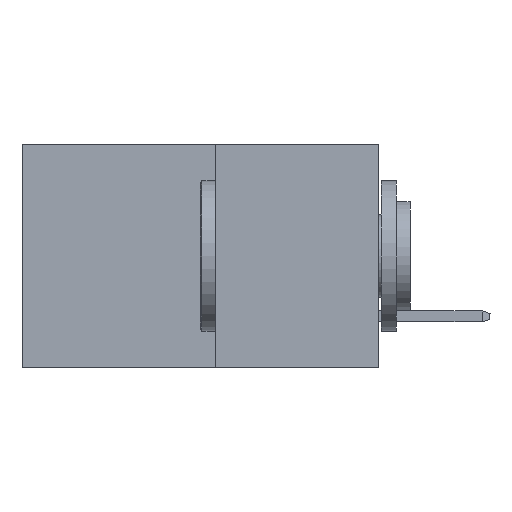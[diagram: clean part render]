
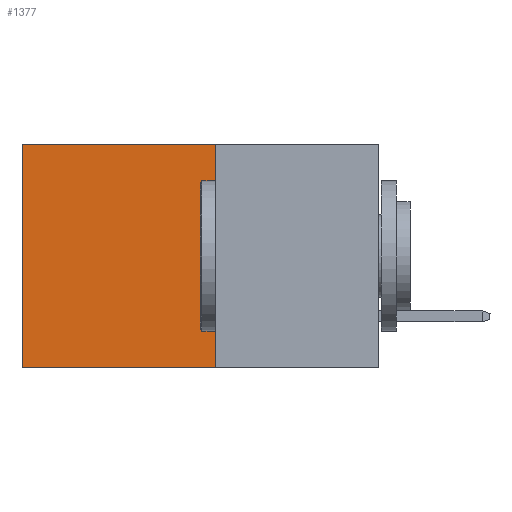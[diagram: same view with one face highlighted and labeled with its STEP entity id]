
A CAD part, left-side view. The second image highlights one B-rep face of the part: STEP entity #1377.
In plain terms, the highlighted planar face has unit normal (-1, 0, 0).
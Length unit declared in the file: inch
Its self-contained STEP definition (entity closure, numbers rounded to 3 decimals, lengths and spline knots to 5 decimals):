
#153 = CARTESIAN_POINT ( 'NONE',  ( 0.277, 0.27, 0. ) ) ;
#684 = VECTOR ( 'NONE', #2647, 39.37008 ) ;
#1377 = ADVANCED_FACE ( 'NONE', ( #27120 ), #6733, .F. ) ;
#1593 = ORIENTED_EDGE ( 'NONE', *, *, #11115, .T. ) ;
#1860 = CARTESIAN_POINT ( 'NONE',  ( 0.277, 0.27, 0. ) ) ;
#2647 = DIRECTION ( 'NONE',  ( 0., 1., 0. ) ) ;
#4749 = VERTEX_POINT ( 'NONE', #24941 ) ;
#5170 = CARTESIAN_POINT ( 'NONE',  ( 0.277, 0.27, -0.37 ) ) ;
#5468 = LINE ( 'NONE', #20682, #18034 ) ;
#6733 = PLANE ( 'NONE',  #15053 ) ;
#8735 = CARTESIAN_POINT ( 'NONE',  ( 0.277, 0.59, -0.37 ) ) ;
#9065 = DIRECTION ( 'NONE',  ( 1., 0., 0. ) ) ;
#9703 = LINE ( 'NONE', #17524, #22224 ) ;
#11115 = EDGE_CURVE ( 'NONE', #4749, #25093, #28056, .T. ) ;
#13111 = VECTOR ( 'NONE', #19176, 39.37008 ) ;
#14018 = LINE ( 'NONE', #153, #684 ) ;
#15053 = AXIS2_PLACEMENT_3D ( 'NONE', #5170, #9065, #28737 ) ;
#15394 = DIRECTION ( 'NONE',  ( 0., 1., 0. ) ) ;
#17524 = CARTESIAN_POINT ( 'NONE',  ( 0.277, 0.27, -0.37 ) ) ;
#18034 = VECTOR ( 'NONE', #18141, 39.37008 ) ;
#18141 = DIRECTION ( 'NONE',  ( 0., 0., -1. ) ) ;
#19176 = DIRECTION ( 'NONE',  ( 0., 0., -1. ) ) ;
#19711 = EDGE_CURVE ( 'NONE', #22144, #25093, #9703, .T. ) ;
#20682 = CARTESIAN_POINT ( 'NONE',  ( 0.277, 0.27, -0.37 ) ) ;
#21290 = ORIENTED_EDGE ( 'NONE', *, *, #19711, .F. ) ;
#22144 = VERTEX_POINT ( 'NONE', #28271 ) ;
#22224 = VECTOR ( 'NONE', #15394, 39.37008 ) ;
#23909 = EDGE_CURVE ( 'NONE', #28597, #22144, #5468, .T. ) ;
#24930 = EDGE_CURVE ( 'NONE', #28597, #4749, #14018, .T. ) ;
#24941 = CARTESIAN_POINT ( 'NONE',  ( 0.277, 0.59, 0. ) ) ;
#25093 = VERTEX_POINT ( 'NONE', #28472 ) ;
#25309 = EDGE_LOOP ( 'NONE', ( #1593, #21290, #27329, #26230 ) ) ;
#26230 = ORIENTED_EDGE ( 'NONE', *, *, #24930, .T. ) ;
#27120 = FACE_OUTER_BOUND ( 'NONE', #25309, .T. ) ;
#27329 = ORIENTED_EDGE ( 'NONE', *, *, #23909, .F. ) ;
#28056 = LINE ( 'NONE', #8735, #13111 ) ;
#28271 = CARTESIAN_POINT ( 'NONE',  ( 0.277, 0.27, -0.37 ) ) ;
#28472 = CARTESIAN_POINT ( 'NONE',  ( 0.277, 0.59, -0.37 ) ) ;
#28597 = VERTEX_POINT ( 'NONE', #1860 ) ;
#28737 = DIRECTION ( 'NONE',  ( 0., 0., -1. ) ) ;
